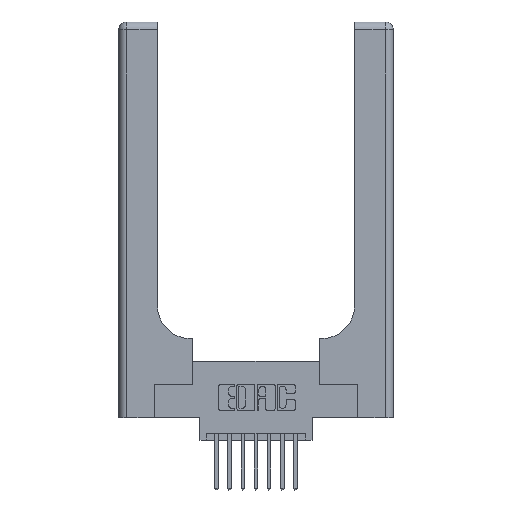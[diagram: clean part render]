
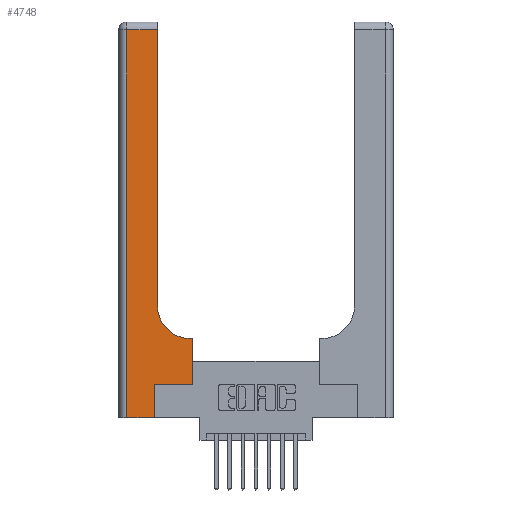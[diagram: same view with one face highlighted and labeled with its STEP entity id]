
A CAD part, top view. The second image highlights one B-rep face of the part: STEP entity #4748.
In plain terms, the highlighted planar face has unit normal (0, 0, 1).
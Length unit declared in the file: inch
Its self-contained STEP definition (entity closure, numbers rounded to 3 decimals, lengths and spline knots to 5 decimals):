
#389 = EDGE_CURVE ( 'NONE', #8636, #3826, #5429, .T. ) ;
#547 = ORIENTED_EDGE ( 'NONE', *, *, #8952, .T. ) ;
#774 = CARTESIAN_POINT ( 'NONE',  ( 0.5585, 0.6, 0.37 ) ) ;
#877 = ORIENTED_EDGE ( 'NONE', *, *, #1449, .T. ) ;
#906 = DIRECTION ( 'NONE',  ( -1., 0., 0. ) ) ;
#938 = CARTESIAN_POINT ( 'NONE',  ( 0., 2.94, 0.37 ) ) ;
#964 = EDGE_CURVE ( 'NONE', #3826, #6977, #7440, .T. ) ;
#1025 = CARTESIAN_POINT ( 'NONE',  ( 0.06, 0., 0.37 ) ) ;
#1224 = VECTOR ( 'NONE', #906, 39.37008 ) ;
#1449 = EDGE_CURVE ( 'NONE', #11932, #9445, #8164, .T. ) ;
#1542 = ORIENTED_EDGE ( 'NONE', *, *, #12924, .T. ) ;
#1796 = VECTOR ( 'NONE', #8742, 39.37008 ) ;
#1870 = VERTEX_POINT ( 'NONE', #3216 ) ;
#2074 = EDGE_CURVE ( 'NONE', #6977, #1870, #4087, .T. ) ;
#3173 = VECTOR ( 'NONE', #11551, 39.37008 ) ;
#3216 = CARTESIAN_POINT ( 'NONE',  ( 0.06, 2.94, 0.37 ) ) ;
#3462 = PLANE ( 'NONE',  #11570 ) ;
#3826 = VERTEX_POINT ( 'NONE', #5333 ) ;
#4087 = LINE ( 'NONE', #938, #1224 ) ;
#4183 = EDGE_LOOP ( 'NONE', ( #10265, #14951, #4286, #9429, #547, #877, #6560, #1542, #14795 ) ) ;
#4279 = VECTOR ( 'NONE', #13607, 39.37008 ) ;
#4286 = ORIENTED_EDGE ( 'NONE', *, *, #9194, .T. ) ;
#4309 = VECTOR ( 'NONE', #10069, 39.37008 ) ;
#4748 = ADVANCED_FACE ( 'NONE', ( #11666 ), #3462, .F. ) ;
#5040 = VERTEX_POINT ( 'NONE', #8833 ) ;
#5333 = CARTESIAN_POINT ( 'NONE',  ( 0.2915, 0.85, 0.37 ) ) ;
#5429 = CIRCLE ( 'NONE', #9642, 0.25 ) ;
#5456 = CARTESIAN_POINT ( 'NONE',  ( 0.2915, 2.94, 0.37 ) ) ;
#5616 = VECTOR ( 'NONE', #7226, 39.37008 ) ;
#6542 = DIRECTION ( 'NONE',  ( 0., -1., 0. ) ) ;
#6560 = ORIENTED_EDGE ( 'NONE', *, *, #12340, .T. ) ;
#6977 = VERTEX_POINT ( 'NONE', #5456 ) ;
#7112 = EDGE_CURVE ( 'NONE', #8781, #5040, #12729, .T. ) ;
#7226 = DIRECTION ( 'NONE',  ( 0., 1., 0. ) ) ;
#7440 = LINE ( 'NONE', #13642, #4279 ) ;
#8164 = LINE ( 'NONE', #8686, #1796 ) ;
#8254 = DIRECTION ( 'NONE',  ( -1., 0., 0. ) ) ;
#8521 = CARTESIAN_POINT ( 'NONE',  ( 0.269, 0., 0.37 ) ) ;
#8636 = VERTEX_POINT ( 'NONE', #10275 ) ;
#8686 = CARTESIAN_POINT ( 'NONE',  ( 0.269, 0.25, 0.37 ) ) ;
#8713 = CARTESIAN_POINT ( 'NONE',  ( 0.269, 0.25, 0.37 ) ) ;
#8742 = DIRECTION ( 'NONE',  ( 1., 0., 0. ) ) ;
#8781 = VERTEX_POINT ( 'NONE', #1025 ) ;
#8833 = CARTESIAN_POINT ( 'NONE',  ( 0.269, 0., 0.37 ) ) ;
#8890 = CARTESIAN_POINT ( 'NONE',  ( 0.06, 3., 0.37 ) ) ;
#8913 = CARTESIAN_POINT ( 'NONE',  ( 0.2915, 0.6, 0.37 ) ) ;
#8952 = EDGE_CURVE ( 'NONE', #5040, #11932, #14520, .T. ) ;
#9194 = EDGE_CURVE ( 'NONE', #1870, #8781, #13957, .T. ) ;
#9429 = ORIENTED_EDGE ( 'NONE', *, *, #7112, .T. ) ;
#9445 = VERTEX_POINT ( 'NONE', #15339 ) ;
#9642 = AXIS2_PLACEMENT_3D ( 'NONE', #11715, #11682, #11667 ) ;
#9737 = DIRECTION ( 'NONE',  ( 0., 1., 0. ) ) ;
#9994 = VERTEX_POINT ( 'NONE', #774 ) ;
#10069 = DIRECTION ( 'NONE',  ( -1., 0., 0. ) ) ;
#10265 = ORIENTED_EDGE ( 'NONE', *, *, #964, .T. ) ;
#10275 = CARTESIAN_POINT ( 'NONE',  ( 0.5415, 0.6, 0.37 ) ) ;
#10778 = VECTOR ( 'NONE', #6542, 39.37008 ) ;
#10791 = CARTESIAN_POINT ( 'NONE',  ( 0.5585, 0.25, 0.37 ) ) ;
#11028 = LINE ( 'NONE', #8913, #4309 ) ;
#11551 = DIRECTION ( 'NONE',  ( 1., 0., 0. ) ) ;
#11570 = AXIS2_PLACEMENT_3D ( 'NONE', #14221, #15397, #8254 ) ;
#11666 = FACE_OUTER_BOUND ( 'NONE', #4183, .T. ) ;
#11667 = DIRECTION ( 'NONE',  ( 1., 0., 0. ) ) ;
#11682 = DIRECTION ( 'NONE',  ( 0., 0., -1. ) ) ;
#11715 = CARTESIAN_POINT ( 'NONE',  ( 0.5415, 0.85, 0.37 ) ) ;
#11932 = VERTEX_POINT ( 'NONE', #8713 ) ;
#12340 = EDGE_CURVE ( 'NONE', #9445, #9994, #15108, .T. ) ;
#12729 = LINE ( 'NONE', #13998, #3173 ) ;
#12924 = EDGE_CURVE ( 'NONE', #9994, #8636, #11028, .T. ) ;
#13607 = DIRECTION ( 'NONE',  ( 0., 1., 0. ) ) ;
#13642 = CARTESIAN_POINT ( 'NONE',  ( 0.2915, 3., 0.37 ) ) ;
#13957 = LINE ( 'NONE', #8890, #10778 ) ;
#13998 = CARTESIAN_POINT ( 'NONE',  ( 0., 0., 0.37 ) ) ;
#14145 = VECTOR ( 'NONE', #9737, 39.37008 ) ;
#14221 = CARTESIAN_POINT ( 'NONE',  ( 0., 3., 0.37 ) ) ;
#14520 = LINE ( 'NONE', #8521, #14145 ) ;
#14795 = ORIENTED_EDGE ( 'NONE', *, *, #389, .T. ) ;
#14951 = ORIENTED_EDGE ( 'NONE', *, *, #2074, .T. ) ;
#15108 = LINE ( 'NONE', #10791, #5616 ) ;
#15339 = CARTESIAN_POINT ( 'NONE',  ( 0.5585, 0.25, 0.37 ) ) ;
#15397 = DIRECTION ( 'NONE',  ( 0., 0., -1. ) ) ;
